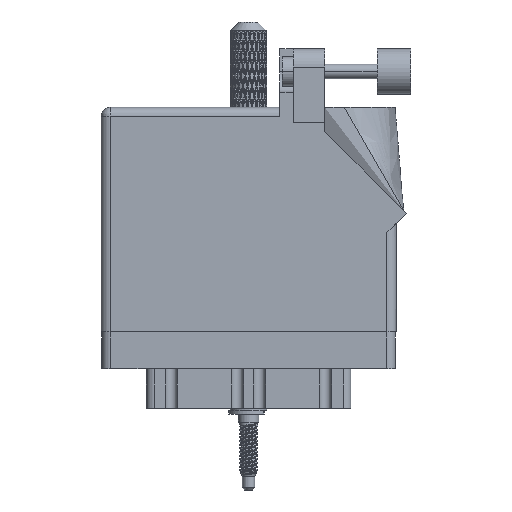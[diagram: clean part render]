
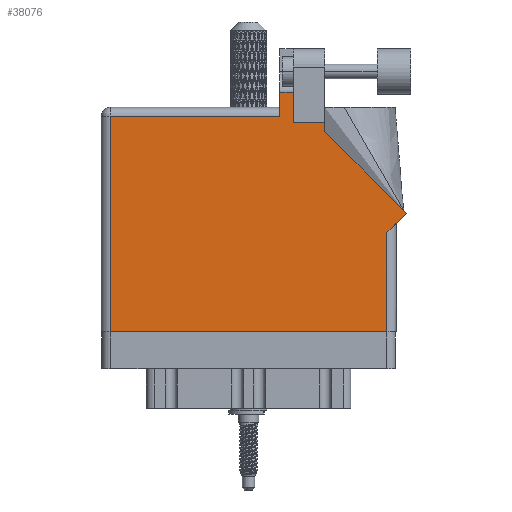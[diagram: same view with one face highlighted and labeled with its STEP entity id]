
A CAD part, front view. The second image highlights one B-rep face of the part: STEP entity #38076.
In plain terms, the highlighted face is planar.
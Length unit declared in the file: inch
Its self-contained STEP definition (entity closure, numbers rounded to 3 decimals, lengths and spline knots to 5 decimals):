
#1003 = ORIENTED_EDGE ( 'NONE', *, *, #59573, .T. ) ;
#1163 = EDGE_CURVE ( 'NONE', #75588, #31541, #37410, .T. ) ;
#1958 = CARTESIAN_POINT ( 'NONE',  ( 1.311, 1.43, 0. ) ) ;
#4212 = ORIENTED_EDGE ( 'NONE', *, *, #47162, .T. ) ;
#4317 = ORIENTED_EDGE ( 'NONE', *, *, #82527, .T. ) ;
#5193 = VECTOR ( 'NONE', #10770, 39.37008 ) ;
#5983 = CARTESIAN_POINT ( 'NONE',  ( 1.64177, 1.6315, 0. ) ) ;
#6605 = DIRECTION ( 'NONE',  ( -1., 0., 0. ) ) ;
#6960 = CARTESIAN_POINT ( 'NONE',  ( 1.948, 0.737, 0. ) ) ;
#7555 = ORIENTED_EDGE ( 'NONE', *, *, #49810, .T. ) ;
#8135 = AXIS2_PLACEMENT_3D ( 'NONE', #62310, #22467, #6605 ) ;
#10770 = DIRECTION ( 'NONE',  ( 0., 1., 0. ) ) ;
#12043 = ORIENTED_EDGE ( 'NONE', *, *, #1163, .T. ) ;
#13194 = VERTEX_POINT ( 'NONE', #88059 ) ;
#13978 = CARTESIAN_POINT ( 'NONE',  ( 0., 1.468, 0. ) ) ;
#14864 = EDGE_CURVE ( 'NONE', #102814, #64555, #17228, .T. ) ;
#15603 = EDGE_CURVE ( 'NONE', #102863, #102814, #95007, .T. ) ;
#17228 = LINE ( 'NONE', #97826, #63585 ) ;
#19739 = CARTESIAN_POINT ( 'NONE',  ( 1.311, 1.43, 0. ) ) ;
#20424 = LINE ( 'NONE', #77712, #25201 ) ;
#20746 = VERTEX_POINT ( 'NONE', #25487 ) ;
#22467 = DIRECTION ( 'NONE',  ( 0., 0., -1. ) ) ;
#22535 = DIRECTION ( 'NONE',  ( -1., 0., 0. ) ) ;
#22812 = VERTEX_POINT ( 'NONE', #33849 ) ;
#25201 = VECTOR ( 'NONE', #61800, 39.37008 ) ;
#25487 = CARTESIAN_POINT ( 'NONE',  ( 1.217, 1.6315, 0. ) ) ;
#26952 = EDGE_CURVE ( 'NONE', #88714, #22812, #62791, .T. ) ;
#27204 = VECTOR ( 'NONE', #50860, 39.37008 ) ;
#30277 = DIRECTION ( 'NONE',  ( 0.707, 0.707, 0. ) ) ;
#31541 = VERTEX_POINT ( 'NONE', #1958 ) ;
#31971 = VECTOR ( 'NONE', #96544, 39.37008 ) ;
#33849 = CARTESIAN_POINT ( 'NONE',  ( 0.062, 1.468, 0. ) ) ;
#37410 = LINE ( 'NONE', #103197, #72247 ) ;
#37758 = DIRECTION ( 'NONE',  ( -1., 0., 0. ) ) ;
#37782 = VECTOR ( 'NONE', #59440, 39.37008 ) ;
#38076 = ADVANCED_FACE ( 'NONE', ( #53797 ), #86167, .F. ) ;
#41153 = CARTESIAN_POINT ( 'NONE',  ( 1.524, 1.36442, 0. ) ) ;
#46122 = ORIENTED_EDGE ( 'NONE', *, *, #66693, .T. ) ;
#46153 = LINE ( 'NONE', #6960, #31971 ) ;
#47162 = EDGE_CURVE ( 'NONE', #13194, #102547, #87098, .T. ) ;
#48511 = EDGE_LOOP ( 'NONE', ( #7555, #82984, #1003, #56628, #46122, #4212, #86658, #51794, #96186, #4317, #12043 ) ) ;
#48981 = VECTOR ( 'NONE', #62738, 39.37008 ) ;
#49810 = EDGE_CURVE ( 'NONE', #31541, #93807, #91865, .T. ) ;
#49957 = CARTESIAN_POINT ( 'NONE',  ( 2.08071, 0.80771, 0. ) ) ;
#50099 = VECTOR ( 'NONE', #30277, 39.37008 ) ;
#50860 = DIRECTION ( 'NONE',  ( 0., -1., 0. ) ) ;
#51794 = ORIENTED_EDGE ( 'NONE', *, *, #15603, .T. ) ;
#53797 = FACE_OUTER_BOUND ( 'NONE', #48511, .T. ) ;
#54719 = CARTESIAN_POINT ( 'NONE',  ( 2.01, 0.737, 0. ) ) ;
#56628 = ORIENTED_EDGE ( 'NONE', *, *, #26952, .T. ) ;
#59440 = DIRECTION ( 'NONE',  ( 0., 1., 0. ) ) ;
#59573 = EDGE_CURVE ( 'NONE', #20746, #88714, #20424, .T. ) ;
#60180 = CARTESIAN_POINT ( 'NONE',  ( 1.217, 1.468, 0. ) ) ;
#61800 = DIRECTION ( 'NONE',  ( 0., -1., 0. ) ) ;
#62211 = LINE ( 'NONE', #5983, #79511 ) ;
#62310 = CARTESIAN_POINT ( 'NONE',  ( 0., 1.53, 0. ) ) ;
#62738 = DIRECTION ( 'NONE',  ( 1., 0., 0. ) ) ;
#62791 = LINE ( 'NONE', #13978, #72708 ) ;
#63585 = VECTOR ( 'NONE', #104754, 39.37008 ) ;
#64029 = EDGE_CURVE ( 'NONE', #93807, #20746, #62211, .T. ) ;
#64555 = VERTEX_POINT ( 'NONE', #41153 ) ;
#66693 = EDGE_CURVE ( 'NONE', #22812, #13194, #99658, .T. ) ;
#67426 = LINE ( 'NONE', #99166, #37782 ) ;
#69218 = CARTESIAN_POINT ( 'NONE',  ( 1.948, 0., 0. ) ) ;
#70233 = DIRECTION ( 'NONE',  ( -1., 0., 0. ) ) ;
#70361 = CARTESIAN_POINT ( 'NONE',  ( 1.524, 1.43, 0. ) ) ;
#72247 = VECTOR ( 'NONE', #22535, 39.37008 ) ;
#72708 = VECTOR ( 'NONE', #70233, 39.37008 ) ;
#74803 = CARTESIAN_POINT ( 'NONE',  ( 0.062, 0., 0. ) ) ;
#75588 = VERTEX_POINT ( 'NONE', #70361 ) ;
#76823 = CARTESIAN_POINT ( 'NONE',  ( 1.311, 1.6315, 0. ) ) ;
#77712 = CARTESIAN_POINT ( 'NONE',  ( 1.217, 1.53, 0. ) ) ;
#79511 = VECTOR ( 'NONE', #37758, 39.37008 ) ;
#82527 = EDGE_CURVE ( 'NONE', #64555, #75588, #67426, .T. ) ;
#82984 = ORIENTED_EDGE ( 'NONE', *, *, #64029, .T. ) ;
#86167 = PLANE ( 'NONE',  #8135 ) ;
#86658 = ORIENTED_EDGE ( 'NONE', *, *, #101591, .T. ) ;
#87098 = LINE ( 'NONE', #91525, #48981 ) ;
#88059 = CARTESIAN_POINT ( 'NONE',  ( 0.062, 0., 0. ) ) ;
#88714 = VERTEX_POINT ( 'NONE', #60180 ) ;
#90308 = CARTESIAN_POINT ( 'NONE',  ( 1.948, 0.675, 0. ) ) ;
#91525 = CARTESIAN_POINT ( 'NONE',  ( 0., 0., 0. ) ) ;
#91865 = LINE ( 'NONE', #19739, #5193 ) ;
#93807 = VERTEX_POINT ( 'NONE', #76823 ) ;
#95007 = LINE ( 'NONE', #54719, #50099 ) ;
#96186 = ORIENTED_EDGE ( 'NONE', *, *, #14864, .T. ) ;
#96544 = DIRECTION ( 'NONE',  ( 0., 1., 0. ) ) ;
#97826 = CARTESIAN_POINT ( 'NONE',  ( 2.08071, 0.80771, 0. ) ) ;
#99166 = CARTESIAN_POINT ( 'NONE',  ( 1.524, 1.36442, 0. ) ) ;
#99658 = LINE ( 'NONE', #74803, #27204 ) ;
#101591 = EDGE_CURVE ( 'NONE', #102547, #102863, #46153, .T. ) ;
#102547 = VERTEX_POINT ( 'NONE', #69218 ) ;
#102814 = VERTEX_POINT ( 'NONE', #49957 ) ;
#102863 = VERTEX_POINT ( 'NONE', #90308 ) ;
#103197 = CARTESIAN_POINT ( 'NONE',  ( 1.524, 1.43, 0. ) ) ;
#104754 = DIRECTION ( 'NONE',  ( -0.707, 0.707, 0. ) ) ;
